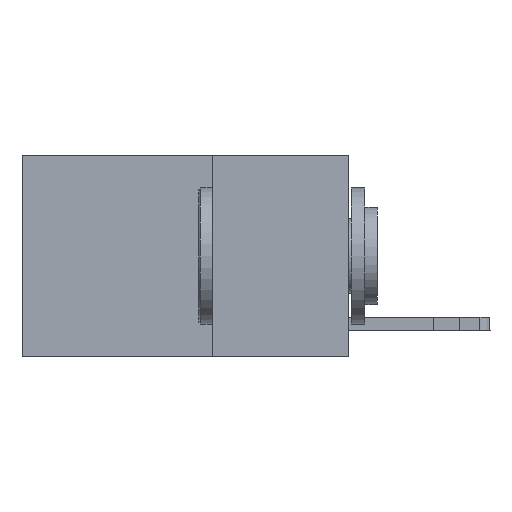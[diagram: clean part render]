
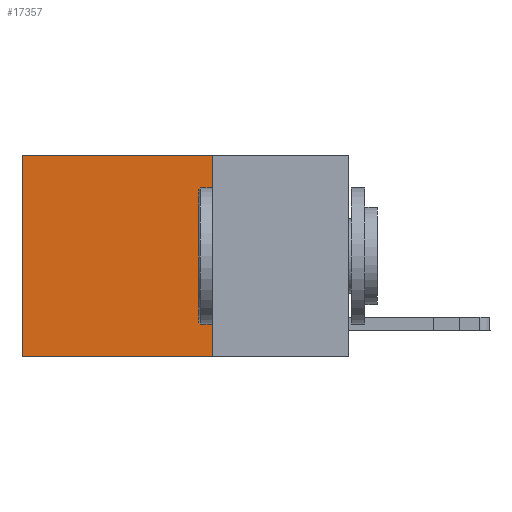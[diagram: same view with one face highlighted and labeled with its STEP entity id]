
A CAD part, left-side view. The second image highlights one B-rep face of the part: STEP entity #17357.
In plain terms, the highlighted planar face has unit normal (-1, 0, 0).
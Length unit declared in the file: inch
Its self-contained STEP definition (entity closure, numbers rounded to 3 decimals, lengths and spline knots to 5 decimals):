
#181 = DIRECTION ( 'NONE',  ( 1., 0., 0. ) ) ;
#197 = ORIENTED_EDGE ( 'NONE', *, *, #12335, .T. ) ;
#443 = VERTEX_POINT ( 'NONE', #14009 ) ;
#485 = CARTESIAN_POINT ( 'NONE',  ( 0.2625, 0.6, 0. ) ) ;
#508 = CARTESIAN_POINT ( 'NONE',  ( 0.2625, 0.25, 0. ) ) ;
#2161 = EDGE_CURVE ( 'NONE', #5461, #6874, #16332, .T. ) ;
#2534 = LINE ( 'NONE', #485, #15567 ) ;
#2836 = PLANE ( 'NONE',  #12937 ) ;
#3080 = EDGE_CURVE ( 'NONE', #4494, #6874, #2534, .T. ) ;
#4494 = VERTEX_POINT ( 'NONE', #10143 ) ;
#5399 = EDGE_LOOP ( 'NONE', ( #13598, #10091, #12967, #197 ) ) ;
#5461 = VERTEX_POINT ( 'NONE', #14606 ) ;
#5526 = DIRECTION ( 'NONE',  ( 0., 0., -1. ) ) ;
#5698 = CARTESIAN_POINT ( 'NONE',  ( 0.2625, 0.25, 0. ) ) ;
#5834 = DIRECTION ( 'NONE',  ( 0., 0., -1. ) ) ;
#5964 = CARTESIAN_POINT ( 'NONE',  ( 0.2625, 0.25, -0.37 ) ) ;
#6106 = VECTOR ( 'NONE', #7525, 39.37008 ) ;
#6874 = VERTEX_POINT ( 'NONE', #15487 ) ;
#7005 = LINE ( 'NONE', #5698, #10270 ) ;
#7525 = DIRECTION ( 'NONE',  ( 0., 1., 0. ) ) ;
#8136 = VECTOR ( 'NONE', #12473, 39.37008 ) ;
#9563 = CARTESIAN_POINT ( 'NONE',  ( 0.2625, 0.25, 0. ) ) ;
#10091 = ORIENTED_EDGE ( 'NONE', *, *, #2161, .F. ) ;
#10143 = CARTESIAN_POINT ( 'NONE',  ( 0.2625, 0.6, 0. ) ) ;
#10270 = VECTOR ( 'NONE', #16408, 39.37008 ) ;
#10762 = EDGE_CURVE ( 'NONE', #443, #5461, #7005, .T. ) ;
#12335 = EDGE_CURVE ( 'NONE', #443, #4494, #15594, .T. ) ;
#12473 = DIRECTION ( 'NONE',  ( 0., 1., 0. ) ) ;
#12937 = AXIS2_PLACEMENT_3D ( 'NONE', #9563, #181, #5526 ) ;
#12967 = ORIENTED_EDGE ( 'NONE', *, *, #10762, .F. ) ;
#13598 = ORIENTED_EDGE ( 'NONE', *, *, #3080, .T. ) ;
#14009 = CARTESIAN_POINT ( 'NONE',  ( 0.2625, 0.25, 0. ) ) ;
#14606 = CARTESIAN_POINT ( 'NONE',  ( 0.2625, 0.25, -0.37 ) ) ;
#14830 = FACE_OUTER_BOUND ( 'NONE', #5399, .T. ) ;
#15487 = CARTESIAN_POINT ( 'NONE',  ( 0.2625, 0.6, -0.37 ) ) ;
#15567 = VECTOR ( 'NONE', #5834, 39.37008 ) ;
#15594 = LINE ( 'NONE', #508, #6106 ) ;
#16332 = LINE ( 'NONE', #5964, #8136 ) ;
#16408 = DIRECTION ( 'NONE',  ( 0., 0., -1. ) ) ;
#17357 = ADVANCED_FACE ( 'NONE', ( #14830 ), #2836, .F. ) ;
